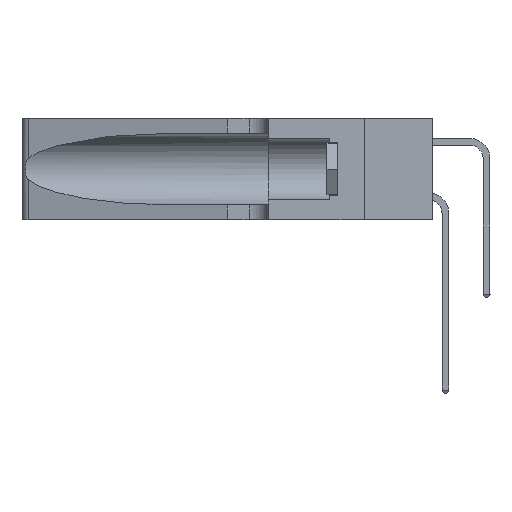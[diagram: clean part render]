
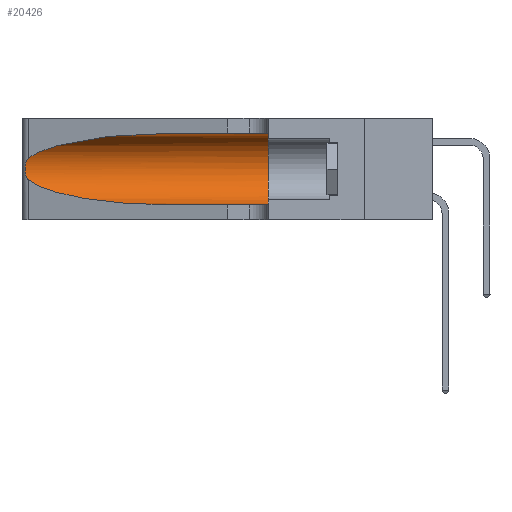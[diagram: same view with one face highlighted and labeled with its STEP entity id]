
A CAD part, left-side view. The second image highlights one B-rep face of the part: STEP entity #20426.
In plain terms, the highlighted cylindrical face has radius 3.308 mm (diameter 6.617 mm), a partial arc.
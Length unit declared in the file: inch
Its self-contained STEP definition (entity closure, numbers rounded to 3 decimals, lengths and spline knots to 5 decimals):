
#606 = CARTESIAN_POINT ( 'NONE',  ( 0.25789, 1.23486, 0.15765 ) ) ;
#842 = CARTESIAN_POINT ( 'NONE',  ( 0.25487, 1.22718, 0.22369 ) ) ;
#1980 = CARTESIAN_POINT ( 'NONE',  ( 0.1305, 0.35, 0.185 ) ) ;
#2866 = AXIS2_PLACEMENT_3D ( 'NONE', #4929, #30776, #33522 ) ;
#3343 = EDGE_CURVE ( 'NONE', #21341, #34423, #19277, .T. ) ;
#3614 = CARTESIAN_POINT ( 'NONE',  ( 0.25854, 1.2359, 0.20912 ) ) ;
#3757 = EDGE_CURVE ( 'NONE', #21341, #34094, #30457, .T. ) ;
#3865 = CARTESIAN_POINT ( 'NONE',  ( 0.25639, 1.23184, 0.21858 ) ) ;
#4929 = CARTESIAN_POINT ( 'NONE',  ( 0.1305, 1.61858, 0.185 ) ) ;
#5074 = VERTEX_POINT ( 'NONE', #5818 ) ;
#5456 = EDGE_LOOP ( 'NONE', ( #5875, #34007, #5839, #33216, #20581, #7715 ) ) ;
#5818 = CARTESIAN_POINT ( 'NONE',  ( 0.1305, 0.72297, 0.05475 ) ) ;
#5839 = ORIENTED_EDGE ( 'NONE', *, *, #21813, .T. ) ;
#5875 = ORIENTED_EDGE ( 'NONE', *, *, #3757, .T. ) ;
#6295 = CARTESIAN_POINT ( 'NONE',  ( 0.26017, 1.23833, 0.17102 ) ) ;
#6425 = CARTESIAN_POINT ( 'NONE',  ( 0.25555, 1.22993, 0.14849 ) ) ;
#6545 = CARTESIAN_POINT ( 'NONE',  ( 0.26075, 1.23896, 0.178 ) ) ;
#6767 = DIRECTION ( 'NONE',  ( 0., -1., 0. ) ) ;
#7715 = ORIENTED_EDGE ( 'NONE', *, *, #3343, .F. ) ;
#8745 = B_SPLINE_CURVE_WITH_KNOTS ( 'NONE', 3,
 ( #842, #19990, #3865, #33363, #3614, #22670, #27922, #6545, #6295, #9266, #606, #22550, #6425, #25006 ),
 .UNSPECIFIED., .F., .F.,
 ( 4, 2, 2, 2, 2, 2, 4 ),
 ( 0., 0.00027, 0.00053, 0.00107, 0.0016, 0.00187, 0.00214 ),
 .UNSPECIFIED. ) ;
#9266 = CARTESIAN_POINT ( 'NONE',  ( 0.25856, 1.23593, 0.16098 ) ) ;
#9405 = CARTESIAN_POINT ( 'NONE',  ( 0.25487, 1.22718, 0.14631 ) ) ;
#9446 = CARTESIAN_POINT ( 'NONE',  ( 0.25487, 1.22718, 0.14631 ) ) ;
#9797 = CARTESIAN_POINT ( 'NONE',  ( 0.1305, 0.72297, 0.05475 ) ) ;
#10141 = EDGE_CURVE ( 'NONE', #34423, #34248, #17365, .T. ) ;
#11597 = CARTESIAN_POINT ( 'NONE',  ( 0.25487, 1.22718, 0.22369 ) ) ;
#12187 = CYLINDRICAL_SURFACE ( 'NONE', #2866, 0.13025 ) ;
#12467 =( BOUNDED_CURVE ( )  B_SPLINE_CURVE ( 3, ( #9446, #17668, #15353, #9797 ),
 .UNSPECIFIED., .F., .F. ) 
 B_SPLINE_CURVE_WITH_KNOTS ( ( 4, 4 ),
 ( 3.44316, 4.71239 ),
 .UNSPECIFIED. ) 
 CURVE ( )  GEOMETRIC_REPRESENTATION_ITEM ( )  RATIONAL_B_SPLINE_CURVE ( ( 1., 0.87, 0.87, 1. ) ) 
 REPRESENTATION_ITEM ( '' )  );
#15122 = VECTOR ( 'NONE', #30547, 39.37008 ) ;
#15257 = CARTESIAN_POINT ( 'NONE',  ( 0.1305, 0.35, 0.31525 ) ) ;
#15353 = CARTESIAN_POINT ( 'NONE',  ( 0.18966, 0.96281, 0.05475 ) ) ;
#15484 = CARTESIAN_POINT ( 'NONE',  ( 0.25487, 1.22718, 0.22369 ) ) ;
#15754 = LINE ( 'NONE', #20082, #32118 ) ;
#15850 = CARTESIAN_POINT ( 'NONE',  ( 0.18966, 0.96281, 0.31525 ) ) ;
#16415 = FACE_OUTER_BOUND ( 'NONE', #5456, .T. ) ;
#17365 = CIRCLE ( 'NONE', #29659, 0.13025 ) ;
#17668 = CARTESIAN_POINT ( 'NONE',  ( 0.2373, 1.15595, 0.08982 ) ) ;
#18080 = CARTESIAN_POINT ( 'NONE',  ( 0.2373, 1.15595, 0.28018 ) ) ;
#18327 = CARTESIAN_POINT ( 'NONE',  ( 0.1305, 0.72297, 0.31525 ) ) ;
#19006 = EDGE_CURVE ( 'NONE', #5074, #34248, #15754, .T. ) ;
#19277 = LINE ( 'NONE', #22728, #15122 ) ;
#19990 = CARTESIAN_POINT ( 'NONE',  ( 0.25555, 1.22994, 0.2215 ) ) ;
#20082 = CARTESIAN_POINT ( 'NONE',  ( 0.1305, 1.61858, 0.05475 ) ) ;
#20426 = ADVANCED_FACE ( 'NONE', ( #16415 ), #12187, .F. ) ;
#20581 = ORIENTED_EDGE ( 'NONE', *, *, #10141, .F. ) ;
#21341 = VERTEX_POINT ( 'NONE', #31174 ) ;
#21813 = EDGE_CURVE ( 'NONE', #23320, #5074, #12467, .T. ) ;
#22550 = CARTESIAN_POINT ( 'NONE',  ( 0.25639, 1.23186, 0.15144 ) ) ;
#22670 = CARTESIAN_POINT ( 'NONE',  ( 0.26018, 1.23835, 0.19895 ) ) ;
#22728 = CARTESIAN_POINT ( 'NONE',  ( 0.1305, 1.61858, 0.31525 ) ) ;
#23278 = EDGE_CURVE ( 'NONE', #34094, #23320, #8745, .T. ) ;
#23320 = VERTEX_POINT ( 'NONE', #9405 ) ;
#25006 = CARTESIAN_POINT ( 'NONE',  ( 0.25487, 1.22718, 0.14631 ) ) ;
#27922 = CARTESIAN_POINT ( 'NONE',  ( 0.26075, 1.23896, 0.19203 ) ) ;
#29123 = DIRECTION ( 'NONE',  ( 0., 1., 0. ) ) ;
#29659 = AXIS2_PLACEMENT_3D ( 'NONE', #1980, #29123, #34803 ) ;
#30457 =( BOUNDED_CURVE ( )  B_SPLINE_CURVE ( 3, ( #18327, #15850, #18080, #15484 ),
 .UNSPECIFIED., .F., .T. ) 
 B_SPLINE_CURVE_WITH_KNOTS ( ( 4, 4 ),
 ( 1.5708, 2.84003 ),
 .UNSPECIFIED. ) 
 CURVE ( )  GEOMETRIC_REPRESENTATION_ITEM ( )  RATIONAL_B_SPLINE_CURVE ( ( 1., 0.87, 0.87, 1. ) ) 
 REPRESENTATION_ITEM ( '' )  );
#30547 = DIRECTION ( 'NONE',  ( 0., -1., 0. ) ) ;
#30776 = DIRECTION ( 'NONE',  ( 0., -1., 0. ) ) ;
#31174 = CARTESIAN_POINT ( 'NONE',  ( 0.1305, 0.72297, 0.31525 ) ) ;
#32118 = VECTOR ( 'NONE', #6767, 39.37008 ) ;
#33216 = ORIENTED_EDGE ( 'NONE', *, *, #19006, .T. ) ;
#33363 = CARTESIAN_POINT ( 'NONE',  ( 0.25787, 1.23484, 0.2124 ) ) ;
#33522 = DIRECTION ( 'NONE',  ( 0., 0., -1. ) ) ;
#33795 = CARTESIAN_POINT ( 'NONE',  ( 0.1305, 0.35, 0.05475 ) ) ;
#34007 = ORIENTED_EDGE ( 'NONE', *, *, #23278, .T. ) ;
#34094 = VERTEX_POINT ( 'NONE', #11597 ) ;
#34248 = VERTEX_POINT ( 'NONE', #33795 ) ;
#34423 = VERTEX_POINT ( 'NONE', #15257 ) ;
#34803 = DIRECTION ( 'NONE',  ( 0., 0., 1. ) ) ;
